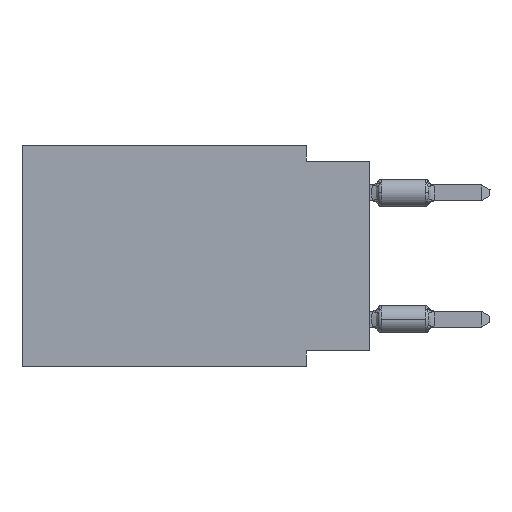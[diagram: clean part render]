
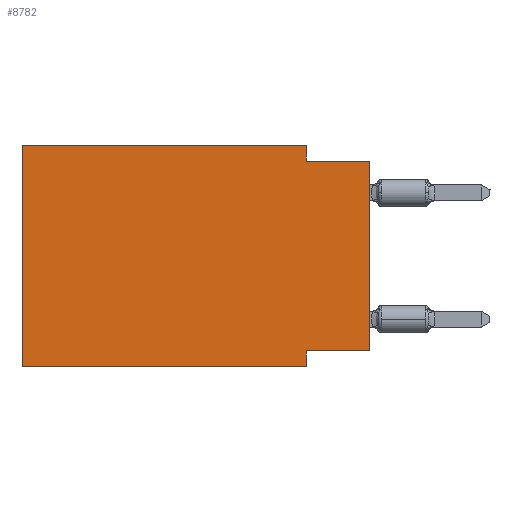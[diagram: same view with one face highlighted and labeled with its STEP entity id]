
A CAD part, left-side view. The second image highlights one B-rep face of the part: STEP entity #8782.
In plain terms, the highlighted planar face has unit normal (-1, 0, 0).
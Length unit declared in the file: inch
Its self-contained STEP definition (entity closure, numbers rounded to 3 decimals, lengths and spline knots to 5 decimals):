
#370 = VERTEX_POINT ( 'NONE', #11199 ) ;
#385 = CARTESIAN_POINT ( 'NONE',  ( 0., 0.55, -0.35 ) ) ;
#517 = VERTEX_POINT ( 'NONE', #15599 ) ;
#1030 = DIRECTION ( 'NONE',  ( 1., 0., 0. ) ) ;
#1179 = PLANE ( 'NONE',  #7722 ) ;
#1481 = VECTOR ( 'NONE', #24847, 39.37008 ) ;
#1580 = DIRECTION ( 'NONE',  ( 0., -1., 0. ) ) ;
#2047 = VECTOR ( 'NONE', #22849, 39.37008 ) ;
#2587 = CARTESIAN_POINT ( 'NONE',  ( 0., 0., 0. ) ) ;
#3558 = ORIENTED_EDGE ( 'NONE', *, *, #10340, .F. ) ;
#3578 = EDGE_CURVE ( 'NONE', #4671, #12032, #22698, .T. ) ;
#4340 = VERTEX_POINT ( 'NONE', #7399 ) ;
#4671 = VERTEX_POINT ( 'NONE', #385 ) ;
#5624 = CARTESIAN_POINT ( 'NONE',  ( 0., 0.55, -0.35 ) ) ;
#5656 = CARTESIAN_POINT ( 'NONE',  ( 0., 0.1, -0.35 ) ) ;
#5666 = CARTESIAN_POINT ( 'NONE',  ( 0., 0., -0.025 ) ) ;
#5821 = DIRECTION ( 'NONE',  ( 0., 1., 0. ) ) ;
#6118 = DIRECTION ( 'NONE',  ( 0., 0., -1. ) ) ;
#7367 = DIRECTION ( 'NONE',  ( 0., 0., 1. ) ) ;
#7399 = CARTESIAN_POINT ( 'NONE',  ( 0., 0.1, 0. ) ) ;
#7565 = VERTEX_POINT ( 'NONE', #5666 ) ;
#7722 = AXIS2_PLACEMENT_3D ( 'NONE', #10722, #1030, #6118 ) ;
#8506 = CARTESIAN_POINT ( 'NONE',  ( 0., 0.1, -0.35 ) ) ;
#8782 = ADVANCED_FACE ( 'NONE', ( #15504 ), #1179, .F. ) ;
#9197 = ORIENTED_EDGE ( 'NONE', *, *, #13223, .F. ) ;
#9965 = ORIENTED_EDGE ( 'NONE', *, *, #3578, .T. ) ;
#10340 = EDGE_CURVE ( 'NONE', #27858, #370, #17526, .T. ) ;
#10722 = CARTESIAN_POINT ( 'NONE',  ( 0., 0.55, 0. ) ) ;
#11199 = CARTESIAN_POINT ( 'NONE',  ( 0., 0.1, -0.325 ) ) ;
#11584 = VECTOR ( 'NONE', #26599, 39.37008 ) ;
#12032 = VERTEX_POINT ( 'NONE', #5656 ) ;
#13223 = EDGE_CURVE ( 'NONE', #18338, #4340, #20114, .T. ) ;
#14300 = EDGE_CURVE ( 'NONE', #27858, #7565, #26476, .T. ) ;
#14679 = ORIENTED_EDGE ( 'NONE', *, *, #28039, .F. ) ;
#15431 = CARTESIAN_POINT ( 'NONE',  ( 0., 0., -0.025 ) ) ;
#15494 = CARTESIAN_POINT ( 'NONE',  ( 0., 0.55, 0. ) ) ;
#15504 = FACE_OUTER_BOUND ( 'NONE', #27551, .T. ) ;
#15599 = CARTESIAN_POINT ( 'NONE',  ( 0., 0.1, -0.025 ) ) ;
#15629 = VECTOR ( 'NONE', #5821, 39.37008 ) ;
#16547 = EDGE_CURVE ( 'NONE', #517, #7565, #26699, .T. ) ;
#17338 = CARTESIAN_POINT ( 'NONE',  ( 0., 0.55, 0. ) ) ;
#17526 = LINE ( 'NONE', #26940, #15629 ) ;
#18324 = EDGE_CURVE ( 'NONE', #4340, #517, #27000, .T. ) ;
#18338 = VERTEX_POINT ( 'NONE', #26552 ) ;
#19252 = ORIENTED_EDGE ( 'NONE', *, *, #16547, .F. ) ;
#19482 = CARTESIAN_POINT ( 'NONE',  ( 0., 0., -0.325 ) ) ;
#20114 = LINE ( 'NONE', #15494, #20120 ) ;
#20120 = VECTOR ( 'NONE', #29081, 39.37008 ) ;
#21164 = VECTOR ( 'NONE', #1580, 39.37008 ) ;
#22698 = LINE ( 'NONE', #5624, #21164 ) ;
#22849 = DIRECTION ( 'NONE',  ( 0., 0., -1. ) ) ;
#24298 = EDGE_CURVE ( 'NONE', #4671, #18338, #29065, .T. ) ;
#24540 = DIRECTION ( 'NONE',  ( 0., 0., -1. ) ) ;
#24624 = VECTOR ( 'NONE', #7367, 39.37008 ) ;
#24688 = CARTESIAN_POINT ( 'NONE',  ( 0., 0.1, 0. ) ) ;
#24847 = DIRECTION ( 'NONE',  ( 0., -1., 0. ) ) ;
#25302 = ORIENTED_EDGE ( 'NONE', *, *, #14300, .T. ) ;
#25545 = ORIENTED_EDGE ( 'NONE', *, *, #24298, .F. ) ;
#26476 = LINE ( 'NONE', #2587, #24624 ) ;
#26552 = CARTESIAN_POINT ( 'NONE',  ( 0., 0.55, 0. ) ) ;
#26599 = DIRECTION ( 'NONE',  ( 0., 0., 1. ) ) ;
#26699 = LINE ( 'NONE', #15431, #1481 ) ;
#26940 = CARTESIAN_POINT ( 'NONE',  ( 0., 0., -0.325 ) ) ;
#27000 = LINE ( 'NONE', #24688, #29604 ) ;
#27551 = EDGE_LOOP ( 'NONE', ( #25302, #19252, #28439, #9197, #25545, #9965, #14679, #3558 ) ) ;
#27858 = VERTEX_POINT ( 'NONE', #19482 ) ;
#28039 = EDGE_CURVE ( 'NONE', #370, #12032, #29940, .T. ) ;
#28439 = ORIENTED_EDGE ( 'NONE', *, *, #18324, .F. ) ;
#29065 = LINE ( 'NONE', #17338, #11584 ) ;
#29081 = DIRECTION ( 'NONE',  ( 0., -1., 0. ) ) ;
#29604 = VECTOR ( 'NONE', #24540, 39.37008 ) ;
#29940 = LINE ( 'NONE', #8506, #2047 ) ;
